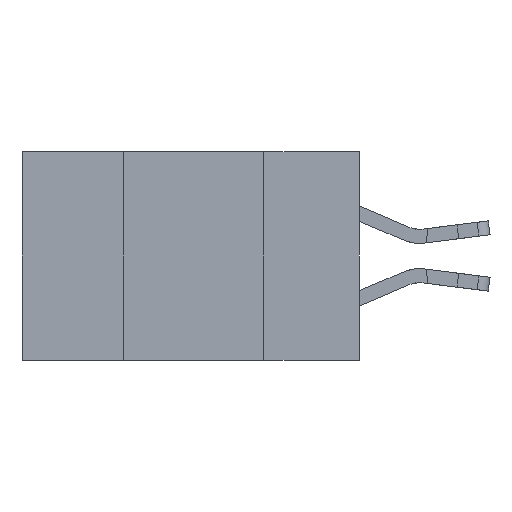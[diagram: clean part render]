
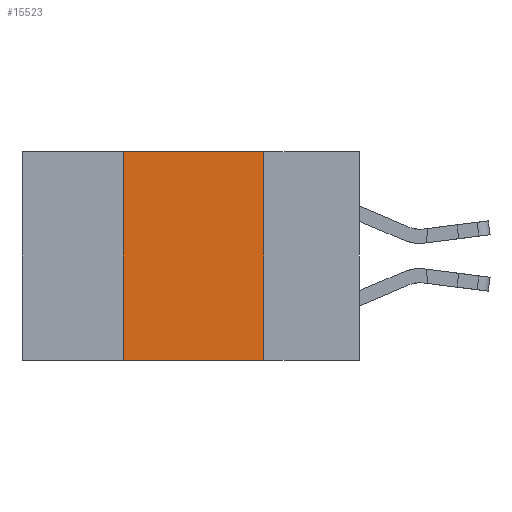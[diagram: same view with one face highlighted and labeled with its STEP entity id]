
A CAD part, left-side view. The second image highlights one B-rep face of the part: STEP entity #15523.
In plain terms, the highlighted planar face has unit normal (-1, 0, 0).
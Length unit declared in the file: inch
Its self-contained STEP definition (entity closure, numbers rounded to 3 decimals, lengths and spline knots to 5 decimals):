
#144 = PLANE ( 'NONE',  #651 ) ;
#651 = AXIS2_PLACEMENT_3D ( 'NONE', #5437, #9377, #14650 ) ;
#2126 = CARTESIAN_POINT ( 'NONE',  ( 0., 0.17, 0. ) ) ;
#3133 = DIRECTION ( 'NONE',  ( 0., -1., 0. ) ) ;
#3245 = CARTESIAN_POINT ( 'NONE',  ( 0., 0.42, 0. ) ) ;
#3402 = VERTEX_POINT ( 'NONE', #12180 ) ;
#5179 = LINE ( 'NONE', #14032, #13820 ) ;
#5437 = CARTESIAN_POINT ( 'NONE',  ( 0., 0.6, 0. ) ) ;
#5699 = CARTESIAN_POINT ( 'NONE',  ( 0., 0.6, 0. ) ) ;
#5976 = DIRECTION ( 'NONE',  ( 0., 0., 1. ) ) ;
#7502 = DIRECTION ( 'NONE',  ( 0., 0., -1. ) ) ;
#7545 = VECTOR ( 'NONE', #10100, 39.37008 ) ;
#7646 = EDGE_CURVE ( 'NONE', #12229, #3402, #15521, .T. ) ;
#8137 = CARTESIAN_POINT ( 'NONE',  ( 0., 0.17, -0.37 ) ) ;
#9198 = LINE ( 'NONE', #9989, #7545 ) ;
#9333 = VECTOR ( 'NONE', #5976, 39.37008 ) ;
#9377 = DIRECTION ( 'NONE',  ( 1., 0., 0. ) ) ;
#9379 = ORIENTED_EDGE ( 'NONE', *, *, #10862, .T. ) ;
#9942 = ORIENTED_EDGE ( 'NONE', *, *, #16769, .F. ) ;
#9989 = CARTESIAN_POINT ( 'NONE',  ( 0., 0.6, -0.37 ) ) ;
#10100 = DIRECTION ( 'NONE',  ( 0., -1., 0. ) ) ;
#10335 = LINE ( 'NONE', #5699, #14644 ) ;
#10849 = VERTEX_POINT ( 'NONE', #2126 ) ;
#10862 = EDGE_CURVE ( 'NONE', #12229, #11843, #9198, .T. ) ;
#11843 = VERTEX_POINT ( 'NONE', #8137 ) ;
#12180 = CARTESIAN_POINT ( 'NONE',  ( 0., 0.42, 0. ) ) ;
#12229 = VERTEX_POINT ( 'NONE', #16901 ) ;
#12852 = ORIENTED_EDGE ( 'NONE', *, *, #13857, .F. ) ;
#13820 = VECTOR ( 'NONE', #7502, 39.37008 ) ;
#13857 = EDGE_CURVE ( 'NONE', #3402, #10849, #10335, .T. ) ;
#14032 = CARTESIAN_POINT ( 'NONE',  ( 0., 0.17, 0. ) ) ;
#14644 = VECTOR ( 'NONE', #3133, 39.37008 ) ;
#14650 = DIRECTION ( 'NONE',  ( 0., 0., -1. ) ) ;
#14963 = ORIENTED_EDGE ( 'NONE', *, *, #7646, .F. ) ;
#15521 = LINE ( 'NONE', #3245, #9333 ) ;
#15523 = ADVANCED_FACE ( 'NONE', ( #16982 ), #144, .F. ) ;
#16769 = EDGE_CURVE ( 'NONE', #10849, #11843, #5179, .T. ) ;
#16901 = CARTESIAN_POINT ( 'NONE',  ( 0., 0.42, -0.37 ) ) ;
#16982 = FACE_OUTER_BOUND ( 'NONE', #16995, .T. ) ;
#16995 = EDGE_LOOP ( 'NONE', ( #9942, #12852, #14963, #9379 ) ) ;
